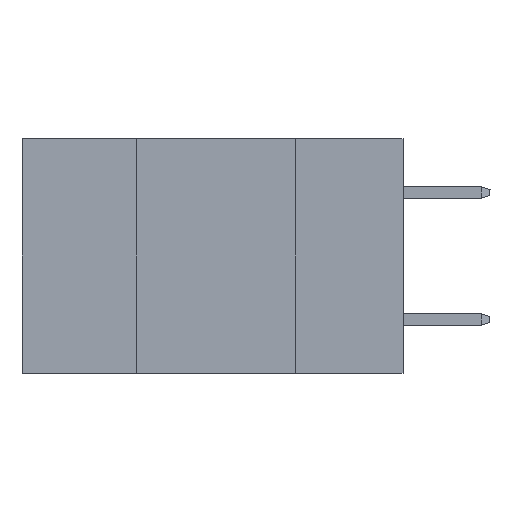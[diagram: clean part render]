
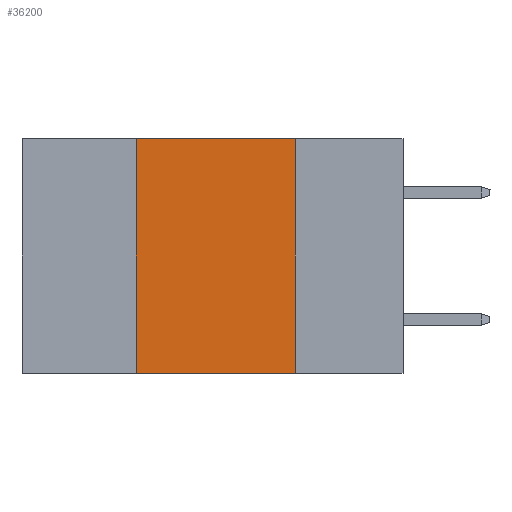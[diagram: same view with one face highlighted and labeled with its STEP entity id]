
A CAD part, left-side view. The second image highlights one B-rep face of the part: STEP entity #36200.
In plain terms, the highlighted planar face has unit normal (-1, 0, 0).
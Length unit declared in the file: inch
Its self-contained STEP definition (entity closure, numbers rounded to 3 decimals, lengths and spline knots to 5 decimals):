
#236 = EDGE_LOOP ( 'NONE', ( #10098, #12423, #10157, #5175 ) ) ;
#749 = DIRECTION ( 'NONE',  ( 0., -1., 0. ) ) ;
#3851 = VECTOR ( 'NONE', #20147, 39.37008 ) ;
#4645 = EDGE_CURVE ( 'NONE', #40793, #33775, #21754, .T. ) ;
#5175 = ORIENTED_EDGE ( 'NONE', *, *, #43950, .T. ) ;
#7564 = FACE_OUTER_BOUND ( 'NONE', #236, .T. ) ;
#9084 = VERTEX_POINT ( 'NONE', #39520 ) ;
#10098 = ORIENTED_EDGE ( 'NONE', *, *, #4645, .F. ) ;
#10157 = ORIENTED_EDGE ( 'NONE', *, *, #20861, .F. ) ;
#12423 = ORIENTED_EDGE ( 'NONE', *, *, #26822, .F. ) ;
#13248 = AXIS2_PLACEMENT_3D ( 'NONE', #22297, #35696, #18862 ) ;
#14126 = CARTESIAN_POINT ( 'NONE',  ( 0., 0.17, -0.37 ) ) ;
#16690 = CARTESIAN_POINT ( 'NONE',  ( 0., 0.6, -0.37 ) ) ;
#18161 = VECTOR ( 'NONE', #749, 39.37008 ) ;
#18862 = DIRECTION ( 'NONE',  ( 0., 0., -1. ) ) ;
#20147 = DIRECTION ( 'NONE',  ( 0., -1., 0. ) ) ;
#20861 = EDGE_CURVE ( 'NONE', #40576, #9084, #37203, .T. ) ;
#21754 = LINE ( 'NONE', #39979, #43641 ) ;
#22297 = CARTESIAN_POINT ( 'NONE',  ( 0., 0.6, 0. ) ) ;
#26822 = EDGE_CURVE ( 'NONE', #9084, #40793, #29924, .T. ) ;
#26929 = VECTOR ( 'NONE', #33523, 39.37008 ) ;
#27070 = CARTESIAN_POINT ( 'NONE',  ( 0., 0.42, 0. ) ) ;
#29924 = LINE ( 'NONE', #42917, #18161 ) ;
#33523 = DIRECTION ( 'NONE',  ( 0., 0., 1. ) ) ;
#33775 = VERTEX_POINT ( 'NONE', #14126 ) ;
#34841 = CARTESIAN_POINT ( 'NONE',  ( 0., 0.17, 0. ) ) ;
#35696 = DIRECTION ( 'NONE',  ( 1., 0., 0. ) ) ;
#35834 = DIRECTION ( 'NONE',  ( 0., 0., -1. ) ) ;
#36200 = ADVANCED_FACE ( 'NONE', ( #7564 ), #43072, .F. ) ;
#37185 = LINE ( 'NONE', #16690, #3851 ) ;
#37203 = LINE ( 'NONE', #27070, #26929 ) ;
#39520 = CARTESIAN_POINT ( 'NONE',  ( 0., 0.42, 0. ) ) ;
#39913 = CARTESIAN_POINT ( 'NONE',  ( 0., 0.42, -0.37 ) ) ;
#39979 = CARTESIAN_POINT ( 'NONE',  ( 0., 0.17, 0. ) ) ;
#40576 = VERTEX_POINT ( 'NONE', #39913 ) ;
#40793 = VERTEX_POINT ( 'NONE', #34841 ) ;
#42917 = CARTESIAN_POINT ( 'NONE',  ( 0., 0.6, 0. ) ) ;
#43072 = PLANE ( 'NONE',  #13248 ) ;
#43641 = VECTOR ( 'NONE', #35834, 39.37008 ) ;
#43950 = EDGE_CURVE ( 'NONE', #40576, #33775, #37185, .T. ) ;
